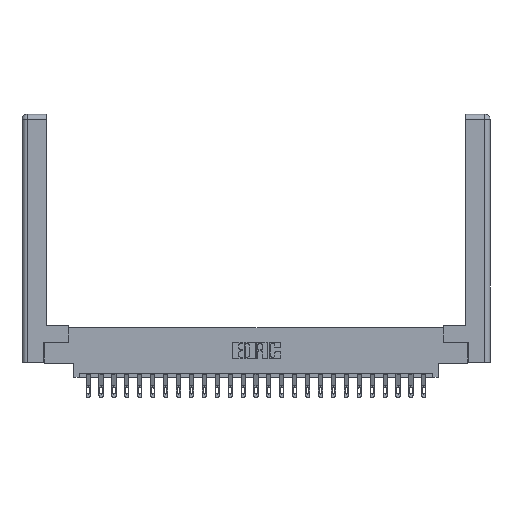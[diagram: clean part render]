
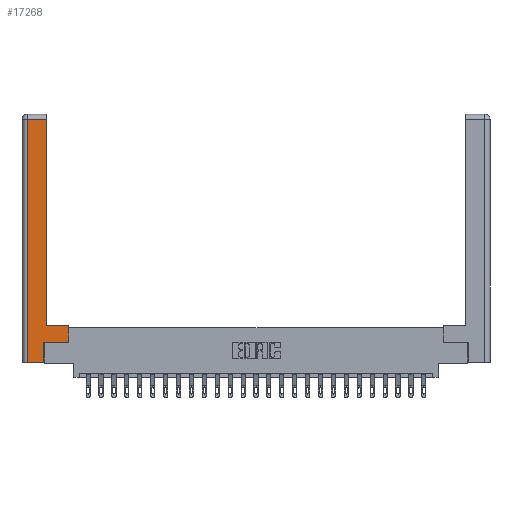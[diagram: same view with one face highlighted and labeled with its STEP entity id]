
A CAD part, top view. The second image highlights one B-rep face of the part: STEP entity #17268.
In plain terms, the highlighted planar face has unit normal (0, 0, 1).
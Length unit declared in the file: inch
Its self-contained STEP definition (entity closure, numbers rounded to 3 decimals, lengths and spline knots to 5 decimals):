
#174 = DIRECTION ( 'NONE',  ( 0., 1., 0. ) ) ;
#1431 = VECTOR ( 'NONE', #24128, 39.37008 ) ;
#1487 = EDGE_CURVE ( 'NONE', #21333, #10467, #24433, .T. ) ;
#1682 = DIRECTION ( 'NONE',  ( 0., 1., 0. ) ) ;
#2039 = PLANE ( 'NONE',  #24658 ) ;
#2129 = CARTESIAN_POINT ( 'NONE',  ( 0., 0., 0. ) ) ;
#2196 = ORIENTED_EDGE ( 'NONE', *, *, #15408, .T. ) ;
#4016 = CARTESIAN_POINT ( 'NONE',  ( 0.265, 0.245, 0. ) ) ;
#4094 = DIRECTION ( 'NONE',  ( 0., -1., 0. ) ) ;
#4137 = VECTOR ( 'NONE', #12271, 39.37008 ) ;
#4149 = CARTESIAN_POINT ( 'NONE',  ( 0.0615, 2.94, 0. ) ) ;
#4164 = EDGE_CURVE ( 'NONE', #9557, #21333, #24886, .T. ) ;
#4481 = CARTESIAN_POINT ( 'NONE',  ( 0.265, 0., 0. ) ) ;
#4883 = LINE ( 'NONE', #4149, #1431 ) ;
#6015 = VECTOR ( 'NONE', #20649, 39.37008 ) ;
#6186 = ORIENTED_EDGE ( 'NONE', *, *, #13424, .T. ) ;
#6194 = CARTESIAN_POINT ( 'NONE',  ( 0.0615, 0., 0. ) ) ;
#6473 = EDGE_CURVE ( 'NONE', #9971, #21465, #17583, .T. ) ;
#7340 = ORIENTED_EDGE ( 'NONE', *, *, #12129, .T. ) ;
#7346 = DIRECTION ( 'NONE',  ( 1., 0., 0. ) ) ;
#7461 = ORIENTED_EDGE ( 'NONE', *, *, #4164, .T. ) ;
#8589 = EDGE_LOOP ( 'NONE', ( #7340, #6186, #7461, #16732, #2196, #16447, #20049, #14799 ) ) ;
#8680 = CARTESIAN_POINT ( 'NONE',  ( 0.565, 0.45, 0. ) ) ;
#9082 = CARTESIAN_POINT ( 'NONE',  ( 0.565, 0.245, 0. ) ) ;
#9557 = VERTEX_POINT ( 'NONE', #24882 ) ;
#9971 = VERTEX_POINT ( 'NONE', #18328 ) ;
#10319 = LINE ( 'NONE', #4016, #20353 ) ;
#10467 = VERTEX_POINT ( 'NONE', #15020 ) ;
#10490 = LINE ( 'NONE', #12619, #6015 ) ;
#11210 = FACE_OUTER_BOUND ( 'NONE', #8589, .T. ) ;
#12058 = CARTESIAN_POINT ( 'NONE',  ( 0.295, 3., 0. ) ) ;
#12129 = EDGE_CURVE ( 'NONE', #21741, #14465, #20336, .T. ) ;
#12271 = DIRECTION ( 'NONE',  ( -1., 0., 0. ) ) ;
#12286 = VECTOR ( 'NONE', #7346, 39.37008 ) ;
#12449 = CARTESIAN_POINT ( 'NONE',  ( 0.295, 0.45, 0. ) ) ;
#12619 = CARTESIAN_POINT ( 'NONE',  ( 0.565, 0.45, 0. ) ) ;
#13424 = EDGE_CURVE ( 'NONE', #14465, #9557, #4883, .T. ) ;
#14465 = VERTEX_POINT ( 'NONE', #23662 ) ;
#14799 = ORIENTED_EDGE ( 'NONE', *, *, #19276, .T. ) ;
#15020 = CARTESIAN_POINT ( 'NONE',  ( 0.265, 0., 0. ) ) ;
#15408 = EDGE_CURVE ( 'NONE', #10467, #9971, #10319, .T. ) ;
#16115 = CARTESIAN_POINT ( 'NONE',  ( 0.0615, 0., 0. ) ) ;
#16447 = ORIENTED_EDGE ( 'NONE', *, *, #6473, .T. ) ;
#16732 = ORIENTED_EDGE ( 'NONE', *, *, #1487, .T. ) ;
#17268 = ADVANCED_FACE ( 'NONE', ( #11210 ), #2039, .F. ) ;
#17583 = LINE ( 'NONE', #21656, #12286 ) ;
#18328 = CARTESIAN_POINT ( 'NONE',  ( 0.265, 0.245, 0. ) ) ;
#19276 = EDGE_CURVE ( 'NONE', #21940, #21741, #20141, .T. ) ;
#19903 = VECTOR ( 'NONE', #4094, 39.37008 ) ;
#19940 = CARTESIAN_POINT ( 'NONE',  ( 0.295, 0.45, 0. ) ) ;
#20024 = VECTOR ( 'NONE', #174, 39.37008 ) ;
#20026 = DIRECTION ( 'NONE',  ( 0., 0., -1. ) ) ;
#20049 = ORIENTED_EDGE ( 'NONE', *, *, #23685, .T. ) ;
#20141 = LINE ( 'NONE', #12449, #4137 ) ;
#20336 = LINE ( 'NONE', #12058, #20024 ) ;
#20353 = VECTOR ( 'NONE', #1682, 39.37008 ) ;
#20649 = DIRECTION ( 'NONE',  ( 0., 1., 0. ) ) ;
#21333 = VERTEX_POINT ( 'NONE', #6194 ) ;
#21465 = VERTEX_POINT ( 'NONE', #9082 ) ;
#21656 = CARTESIAN_POINT ( 'NONE',  ( 0.565, 0.245, 0. ) ) ;
#21741 = VERTEX_POINT ( 'NONE', #19940 ) ;
#21940 = VERTEX_POINT ( 'NONE', #8680 ) ;
#22205 = DIRECTION ( 'NONE',  ( -1., 0., 0. ) ) ;
#23662 = CARTESIAN_POINT ( 'NONE',  ( 0.295, 2.94, 0. ) ) ;
#23685 = EDGE_CURVE ( 'NONE', #21465, #21940, #10490, .T. ) ;
#24128 = DIRECTION ( 'NONE',  ( -1., 0., 0. ) ) ;
#24433 = LINE ( 'NONE', #4481, #24760 ) ;
#24468 = DIRECTION ( 'NONE',  ( 1., 0., 0. ) ) ;
#24658 = AXIS2_PLACEMENT_3D ( 'NONE', #2129, #20026, #22205 ) ;
#24760 = VECTOR ( 'NONE', #24468, 39.37008 ) ;
#24882 = CARTESIAN_POINT ( 'NONE',  ( 0.0615, 2.94, 0. ) ) ;
#24886 = LINE ( 'NONE', #16115, #19903 ) ;
